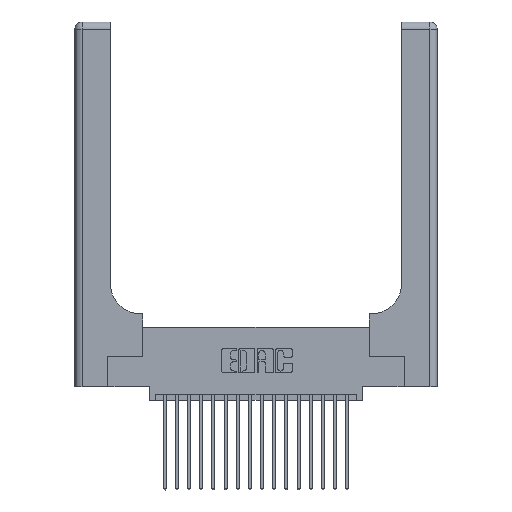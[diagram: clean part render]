
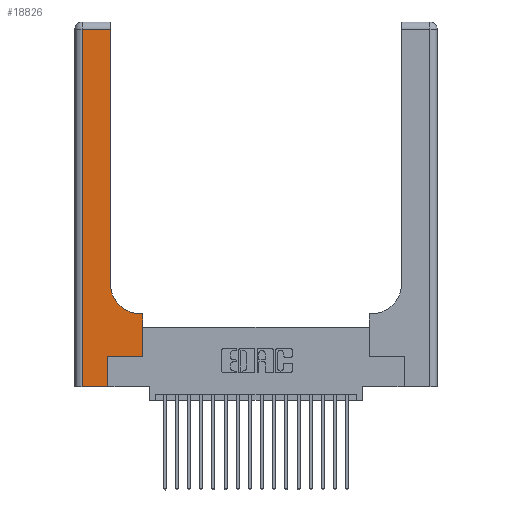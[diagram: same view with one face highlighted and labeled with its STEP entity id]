
A CAD part, top view. The second image highlights one B-rep face of the part: STEP entity #18826.
In plain terms, the highlighted planar face has unit normal (0, 0, 1).
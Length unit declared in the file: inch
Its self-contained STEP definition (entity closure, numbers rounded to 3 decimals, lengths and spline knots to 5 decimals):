
#362 = VERTEX_POINT ( 'NONE', #4381 ) ;
#403 = VECTOR ( 'NONE', #14507, 39.37008 ) ;
#1176 = DIRECTION ( 'NONE',  ( 1., 0., 0. ) ) ;
#1307 = EDGE_CURVE ( 'NONE', #6617, #17800, #20249, .T. ) ;
#1645 = CARTESIAN_POINT ( 'NONE',  ( 0.2915, 0.6, 0.37 ) ) ;
#1648 = CARTESIAN_POINT ( 'NONE',  ( 0.06, 0., 0.37 ) ) ;
#1753 = EDGE_CURVE ( 'NONE', #3923, #5563, #15573, .T. ) ;
#1941 = VECTOR ( 'NONE', #18383, 39.37008 ) ;
#2104 = ORIENTED_EDGE ( 'NONE', *, *, #1753, .T. ) ;
#2248 = DIRECTION ( 'NONE',  ( 1., 0., 0. ) ) ;
#2760 = CARTESIAN_POINT ( 'NONE',  ( 0.5585, 0.6, 0.37 ) ) ;
#3589 = VECTOR ( 'NONE', #15820, 39.37008 ) ;
#3780 = LINE ( 'NONE', #20755, #7897 ) ;
#3923 = VERTEX_POINT ( 'NONE', #11271 ) ;
#3972 = VECTOR ( 'NONE', #1176, 39.37008 ) ;
#4040 = CARTESIAN_POINT ( 'NONE',  ( 0.269, 0., 0.37 ) ) ;
#4097 = CARTESIAN_POINT ( 'NONE',  ( 0., 3., 0.37 ) ) ;
#4381 = CARTESIAN_POINT ( 'NONE',  ( 0.269, 0.25, 0.37 ) ) ;
#4743 = DIRECTION ( 'NONE',  ( 0., 0., -1. ) ) ;
#4948 = DIRECTION ( 'NONE',  ( -1., 0., 0. ) ) ;
#5202 = CARTESIAN_POINT ( 'NONE',  ( 0.2915, 2.94, 0.37 ) ) ;
#5563 = VERTEX_POINT ( 'NONE', #1648 ) ;
#6617 = VERTEX_POINT ( 'NONE', #18468 ) ;
#6941 = LINE ( 'NONE', #12466, #3589 ) ;
#7053 = EDGE_CURVE ( 'NONE', #20348, #3923, #17945, .T. ) ;
#7308 = PLANE ( 'NONE',  #7371 ) ;
#7371 = AXIS2_PLACEMENT_3D ( 'NONE', #4097, #17358, #20481 ) ;
#7472 = DIRECTION ( 'NONE',  ( 0., -1., 0. ) ) ;
#7481 = ORIENTED_EDGE ( 'NONE', *, *, #12117, .T. ) ;
#7650 = EDGE_CURVE ( 'NONE', #18232, #20348, #3780, .T. ) ;
#7897 = VECTOR ( 'NONE', #9125, 39.37008 ) ;
#8253 = EDGE_CURVE ( 'NONE', #17800, #11592, #18434, .T. ) ;
#8556 = EDGE_CURVE ( 'NONE', #362, #6617, #13016, .T. ) ;
#8756 = CARTESIAN_POINT ( 'NONE',  ( 0.06, 3., 0.37 ) ) ;
#9125 = DIRECTION ( 'NONE',  ( 0., 1., 0. ) ) ;
#9723 = CARTESIAN_POINT ( 'NONE',  ( 0.5415, 0.85, 0.37 ) ) ;
#10108 = CARTESIAN_POINT ( 'NONE',  ( 0.5585, 0.25, 0.37 ) ) ;
#10769 = CARTESIAN_POINT ( 'NONE',  ( 0.2915, 0.85, 0.37 ) ) ;
#10799 = CARTESIAN_POINT ( 'NONE',  ( 0.5415, 0.6, 0.37 ) ) ;
#11271 = CARTESIAN_POINT ( 'NONE',  ( 0.06, 2.94, 0.37 ) ) ;
#11407 = ORIENTED_EDGE ( 'NONE', *, *, #8253, .T. ) ;
#11592 = VERTEX_POINT ( 'NONE', #10799 ) ;
#11744 = VECTOR ( 'NONE', #4948, 39.37008 ) ;
#12117 = EDGE_CURVE ( 'NONE', #12523, #362, #6941, .T. ) ;
#12173 = ORIENTED_EDGE ( 'NONE', *, *, #7650, .T. ) ;
#12384 = ORIENTED_EDGE ( 'NONE', *, *, #14988, .T. ) ;
#12466 = CARTESIAN_POINT ( 'NONE',  ( 0.269, 0., 0.37 ) ) ;
#12474 = CARTESIAN_POINT ( 'NONE',  ( 0.269, 0.25, 0.37 ) ) ;
#12523 = VERTEX_POINT ( 'NONE', #4040 ) ;
#13016 = LINE ( 'NONE', #12474, #3972 ) ;
#13629 = ORIENTED_EDGE ( 'NONE', *, *, #7053, .T. ) ;
#13681 = EDGE_CURVE ( 'NONE', #11592, #18232, #14546, .T. ) ;
#14202 = LINE ( 'NONE', #18741, #20400 ) ;
#14507 = DIRECTION ( 'NONE',  ( -1., 0., 0. ) ) ;
#14546 = CIRCLE ( 'NONE', #16154, 0.25 ) ;
#14988 = EDGE_CURVE ( 'NONE', #5563, #12523, #14202, .T. ) ;
#15359 = FACE_OUTER_BOUND ( 'NONE', #20086, .T. ) ;
#15573 = LINE ( 'NONE', #8756, #18686 ) ;
#15820 = DIRECTION ( 'NONE',  ( 0., 1., 0. ) ) ;
#16154 = AXIS2_PLACEMENT_3D ( 'NONE', #9723, #4743, #21281 ) ;
#17358 = DIRECTION ( 'NONE',  ( 0., 0., -1. ) ) ;
#17800 = VERTEX_POINT ( 'NONE', #2760 ) ;
#17945 = LINE ( 'NONE', #20844, #403 ) ;
#18232 = VERTEX_POINT ( 'NONE', #10769 ) ;
#18383 = DIRECTION ( 'NONE',  ( 0., 1., 0. ) ) ;
#18434 = LINE ( 'NONE', #1645, #11744 ) ;
#18468 = CARTESIAN_POINT ( 'NONE',  ( 0.5585, 0.25, 0.37 ) ) ;
#18686 = VECTOR ( 'NONE', #7472, 39.37008 ) ;
#18741 = CARTESIAN_POINT ( 'NONE',  ( 0., 0., 0.37 ) ) ;
#18826 = ADVANCED_FACE ( 'NONE', ( #15359 ), #7308, .F. ) ;
#19730 = ORIENTED_EDGE ( 'NONE', *, *, #8556, .T. ) ;
#20086 = EDGE_LOOP ( 'NONE', ( #12173, #13629, #2104, #12384, #7481, #19730, #20694, #11407, #20496 ) ) ;
#20249 = LINE ( 'NONE', #10108, #1941 ) ;
#20348 = VERTEX_POINT ( 'NONE', #5202 ) ;
#20400 = VECTOR ( 'NONE', #2248, 39.37008 ) ;
#20481 = DIRECTION ( 'NONE',  ( -1., 0., 0. ) ) ;
#20496 = ORIENTED_EDGE ( 'NONE', *, *, #13681, .T. ) ;
#20694 = ORIENTED_EDGE ( 'NONE', *, *, #1307, .T. ) ;
#20755 = CARTESIAN_POINT ( 'NONE',  ( 0.2915, 3., 0.37 ) ) ;
#20844 = CARTESIAN_POINT ( 'NONE',  ( 0., 2.94, 0.37 ) ) ;
#21281 = DIRECTION ( 'NONE',  ( 1., 0., 0. ) ) ;
